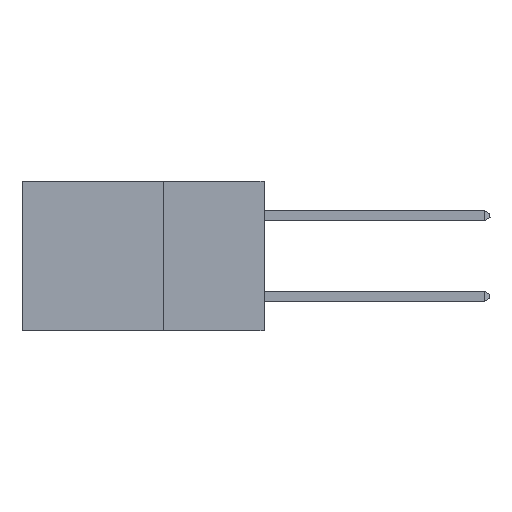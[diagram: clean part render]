
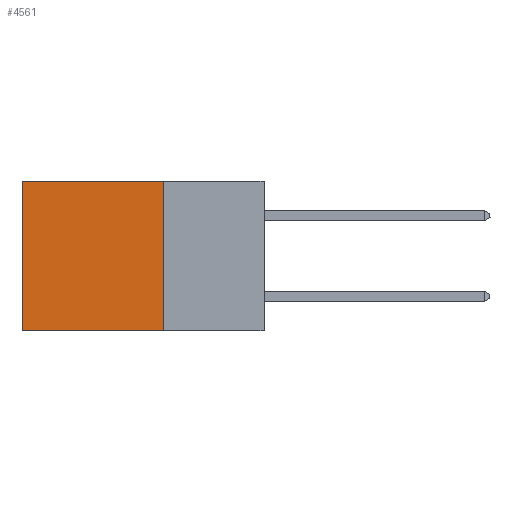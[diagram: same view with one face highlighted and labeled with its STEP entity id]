
A CAD part, left-side view. The second image highlights one B-rep face of the part: STEP entity #4561.
In plain terms, the highlighted planar face has unit normal (-1, 0, 0).
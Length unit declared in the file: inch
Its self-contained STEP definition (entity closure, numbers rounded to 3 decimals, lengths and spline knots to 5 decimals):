
#510 = PLANE ( 'NONE',  #2441 ) ;
#890 = LINE ( 'NONE', #13281, #9110 ) ;
#1325 = ORIENTED_EDGE ( 'NONE', *, *, #3061, .T. ) ;
#2437 = DIRECTION ( 'NONE',  ( 0., 0., -1. ) ) ;
#2441 = AXIS2_PLACEMENT_3D ( 'NONE', #12206, #5834, #3814 ) ;
#3061 = EDGE_CURVE ( 'NONE', #5148, #5359, #10784, .T. ) ;
#3111 = VECTOR ( 'NONE', #4939, 39.37008 ) ;
#3814 = DIRECTION ( 'NONE',  ( 0., 0., -1. ) ) ;
#3918 = EDGE_CURVE ( 'NONE', #5148, #7088, #7383, .T. ) ;
#4468 = CARTESIAN_POINT ( 'NONE',  ( 0.298, 0.25, 0. ) ) ;
#4561 = ADVANCED_FACE ( 'NONE', ( #9067 ), #510, .F. ) ;
#4939 = DIRECTION ( 'NONE',  ( 0., 1., 0. ) ) ;
#5002 = ORIENTED_EDGE ( 'NONE', *, *, #3918, .F. ) ;
#5148 = VERTEX_POINT ( 'NONE', #12584 ) ;
#5359 = VERTEX_POINT ( 'NONE', #7051 ) ;
#5834 = DIRECTION ( 'NONE',  ( 1., 0., 0. ) ) ;
#6786 = ORIENTED_EDGE ( 'NONE', *, *, #9291, .T. ) ;
#6845 = DIRECTION ( 'NONE',  ( 0., 0., -1. ) ) ;
#7051 = CARTESIAN_POINT ( 'NONE',  ( 0.298, 0.6, 0. ) ) ;
#7088 = VERTEX_POINT ( 'NONE', #13620 ) ;
#7203 = VECTOR ( 'NONE', #2437, 39.37008 ) ;
#7383 = LINE ( 'NONE', #4468, #7203 ) ;
#7624 = ORIENTED_EDGE ( 'NONE', *, *, #13798, .F. ) ;
#7730 = VECTOR ( 'NONE', #10178, 39.37008 ) ;
#7962 = CARTESIAN_POINT ( 'NONE',  ( 0.298, 0.25, 0. ) ) ;
#9037 = CARTESIAN_POINT ( 'NONE',  ( 0.298, 0.25, -0.37 ) ) ;
#9067 = FACE_OUTER_BOUND ( 'NONE', #11689, .T. ) ;
#9110 = VECTOR ( 'NONE', #6845, 39.37008 ) ;
#9291 = EDGE_CURVE ( 'NONE', #5359, #11544, #890, .T. ) ;
#9951 = LINE ( 'NONE', #9037, #3111 ) ;
#10178 = DIRECTION ( 'NONE',  ( 0., 1., 0. ) ) ;
#10742 = CARTESIAN_POINT ( 'NONE',  ( 0.298, 0.6, -0.37 ) ) ;
#10784 = LINE ( 'NONE', #7962, #7730 ) ;
#11544 = VERTEX_POINT ( 'NONE', #10742 ) ;
#11689 = EDGE_LOOP ( 'NONE', ( #6786, #7624, #5002, #1325 ) ) ;
#12206 = CARTESIAN_POINT ( 'NONE',  ( 0.298, 0.25, 0. ) ) ;
#12584 = CARTESIAN_POINT ( 'NONE',  ( 0.298, 0.25, 0. ) ) ;
#13281 = CARTESIAN_POINT ( 'NONE',  ( 0.298, 0.6, 0. ) ) ;
#13620 = CARTESIAN_POINT ( 'NONE',  ( 0.298, 0.25, -0.37 ) ) ;
#13798 = EDGE_CURVE ( 'NONE', #7088, #11544, #9951, .T. ) ;
